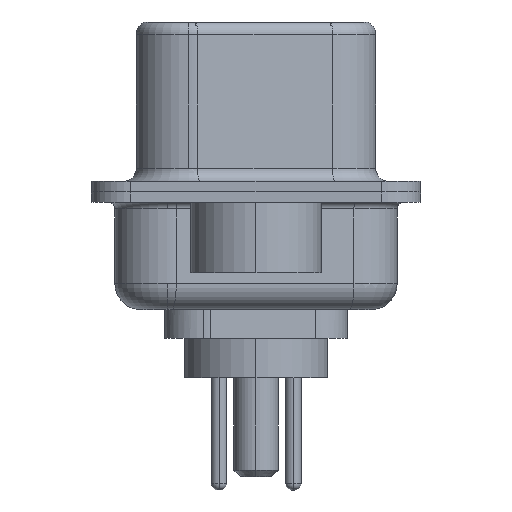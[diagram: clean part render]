
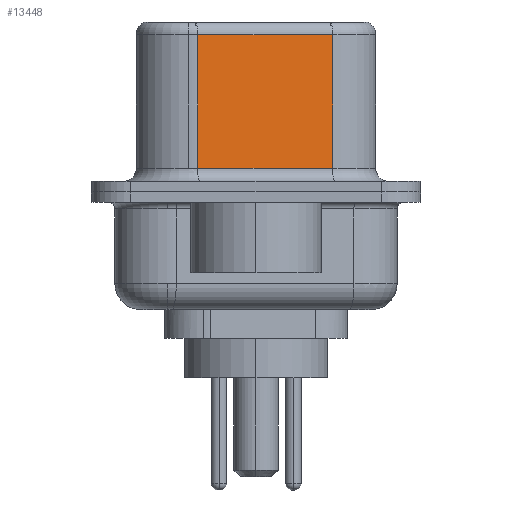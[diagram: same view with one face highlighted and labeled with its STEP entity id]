
A CAD part, left-side view. The second image highlights one B-rep face of the part: STEP entity #13448.
In plain terms, the highlighted planar face has unit normal (-0.985, -0.174, 0).
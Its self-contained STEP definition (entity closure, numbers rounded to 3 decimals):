
#2042 = ORIENTED_EDGE ( 'NONE', *, *, #22823, .T. ) ;
#2591 = DIRECTION ( 'NONE',  ( 0.174, -0.985, 0. ) ) ;
#6486 = EDGE_CURVE ( 'NONE', #17171, #21929, #22149, .T. ) ;
#8369 = CARTESIAN_POINT ( 'NONE',  ( 3.67, 2.233, 6.52 ) ) ;
#8619 = FACE_OUTER_BOUND ( 'NONE', #12960, .T. ) ;
#8693 = VERTEX_POINT ( 'NONE', #16592 ) ;
#10254 = VECTOR ( 'NONE', #2591, 1000. ) ;
#10346 = DIRECTION ( 'NONE',  ( 0., 0., -1. ) ) ;
#11369 = CARTESIAN_POINT ( 'NONE',  ( 4.58, -2.927, 6.52 ) ) ;
#11453 = DIRECTION ( 'NONE',  ( -0.174, 0.985, 0. ) ) ;
#12101 = CARTESIAN_POINT ( 'NONE',  ( 4.58, -2.927, 6.02 ) ) ;
#12523 = CARTESIAN_POINT ( 'NONE',  ( 4.58, -2.927, 6.52 ) ) ;
#12960 = EDGE_LOOP ( 'NONE', ( #21233, #22684, #2042, #22211 ) ) ;
#13448 = ADVANCED_FACE ( 'NONE', ( #8619 ), #17425, .F. ) ;
#14038 = CARTESIAN_POINT ( 'NONE',  ( 3.67, 2.233, 0.9 ) ) ;
#14919 = CARTESIAN_POINT ( 'NONE',  ( 4.58, -2.927, 0.9 ) ) ;
#14971 = LINE ( 'NONE', #8369, #24974 ) ;
#15463 = EDGE_CURVE ( 'NONE', #17171, #8693, #15493, .T. ) ;
#15493 = LINE ( 'NONE', #12101, #25477 ) ;
#15659 = LINE ( 'NONE', #21866, #10254 ) ;
#16592 = CARTESIAN_POINT ( 'NONE',  ( 3.67, 2.233, 6.02 ) ) ;
#16857 = VECTOR ( 'NONE', #21734, 1000. ) ;
#17171 = VERTEX_POINT ( 'NONE', #20067 ) ;
#17425 = PLANE ( 'NONE',  #18735 ) ;
#18735 = AXIS2_PLACEMENT_3D ( 'NONE', #11369, #23438, #11453 ) ;
#20067 = CARTESIAN_POINT ( 'NONE',  ( 4.58, -2.927, 6.02 ) ) ;
#21233 = ORIENTED_EDGE ( 'NONE', *, *, #6486, .F. ) ;
#21734 = DIRECTION ( 'NONE',  ( 0., 0., -1. ) ) ;
#21866 = CARTESIAN_POINT ( 'NONE',  ( 4.58, -2.927, 0.9 ) ) ;
#21929 = VERTEX_POINT ( 'NONE', #14919 ) ;
#22149 = LINE ( 'NONE', #12523, #16857 ) ;
#22211 = ORIENTED_EDGE ( 'NONE', *, *, #22231, .T. ) ;
#22231 = EDGE_CURVE ( 'NONE', #25992, #21929, #15659, .T. ) ;
#22684 = ORIENTED_EDGE ( 'NONE', *, *, #15463, .T. ) ;
#22823 = EDGE_CURVE ( 'NONE', #8693, #25992, #14971, .T. ) ;
#23438 = DIRECTION ( 'NONE',  ( 0.985, 0.174, 0. ) ) ;
#24088 = DIRECTION ( 'NONE',  ( -0.174, 0.985, 0. ) ) ;
#24974 = VECTOR ( 'NONE', #10346, 1000. ) ;
#25477 = VECTOR ( 'NONE', #24088, 1000. ) ;
#25992 = VERTEX_POINT ( 'NONE', #14038 ) ;
